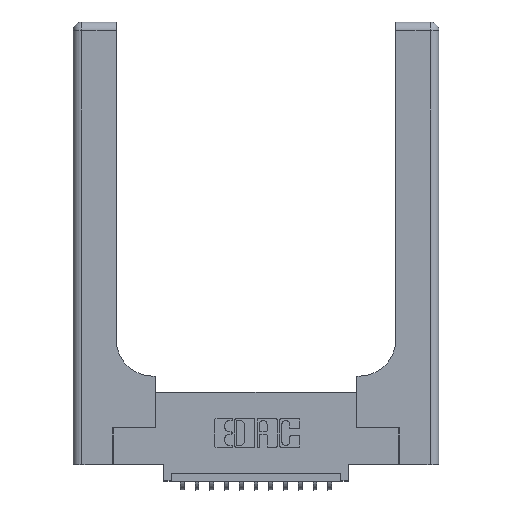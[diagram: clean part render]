
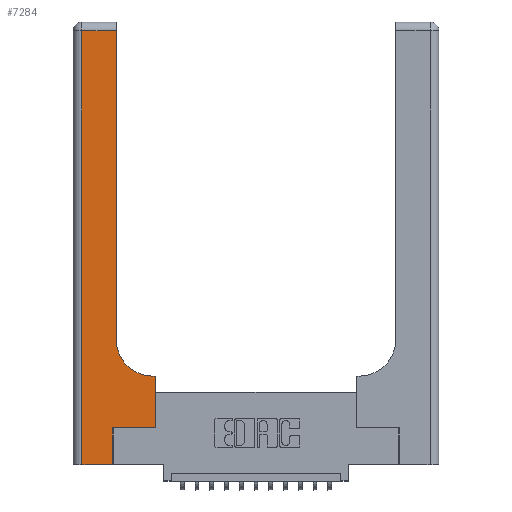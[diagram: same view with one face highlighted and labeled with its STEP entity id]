
A CAD part, top view. The second image highlights one B-rep face of the part: STEP entity #7284.
In plain terms, the highlighted planar face has unit normal (0, 0, 1).
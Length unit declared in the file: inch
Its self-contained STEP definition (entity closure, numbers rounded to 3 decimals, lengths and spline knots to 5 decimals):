
#364 = CARTESIAN_POINT ( 'NONE',  ( 0.5415, 0.6, 0.37 ) ) ;
#785 = LINE ( 'NONE', #7265, #16492 ) ;
#887 = PLANE ( 'NONE',  #12896 ) ;
#1168 = EDGE_CURVE ( 'NONE', #5786, #10817, #5790, .T. ) ;
#1762 = VERTEX_POINT ( 'NONE', #364 ) ;
#1846 = DIRECTION ( 'NONE',  ( -1., 0., 0. ) ) ;
#2134 = CARTESIAN_POINT ( 'NONE',  ( 0., 3., 0.37 ) ) ;
#2148 = VERTEX_POINT ( 'NONE', #14858 ) ;
#2368 = CARTESIAN_POINT ( 'NONE',  ( 0.5585, 0.6, 0.37 ) ) ;
#2928 = DIRECTION ( 'NONE',  ( 1., 0., 0. ) ) ;
#3011 = VERTEX_POINT ( 'NONE', #17585 ) ;
#3127 = ORIENTED_EDGE ( 'NONE', *, *, #14056, .T. ) ;
#3172 = ORIENTED_EDGE ( 'NONE', *, *, #12631, .T. ) ;
#3274 = EDGE_LOOP ( 'NONE', ( #9710, #10301, #8726, #12292, #3172, #3725, #3127, #12026, #11524 ) ) ;
#3385 = DIRECTION ( 'NONE',  ( 0., -1., 0. ) ) ;
#3417 = CARTESIAN_POINT ( 'NONE',  ( 0.2915, 3., 0.37 ) ) ;
#3511 = EDGE_CURVE ( 'NONE', #15576, #5786, #11844, .T. ) ;
#3723 = DIRECTION ( 'NONE',  ( 0., 0., -1. ) ) ;
#3725 = ORIENTED_EDGE ( 'NONE', *, *, #15853, .T. ) ;
#3999 = VECTOR ( 'NONE', #8316, 39.37008 ) ;
#4327 = CARTESIAN_POINT ( 'NONE',  ( 0., 0., 0.37 ) ) ;
#4701 = CARTESIAN_POINT ( 'NONE',  ( 0.2915, 2.94, 0.37 ) ) ;
#4728 = VECTOR ( 'NONE', #15748, 39.37008 ) ;
#5308 = DIRECTION ( 'NONE',  ( 0., 0., -1. ) ) ;
#5344 = VECTOR ( 'NONE', #11607, 39.37008 ) ;
#5596 = LINE ( 'NONE', #11633, #15741 ) ;
#5786 = VERTEX_POINT ( 'NONE', #4701 ) ;
#5790 = LINE ( 'NONE', #8971, #4728 ) ;
#6534 = FACE_OUTER_BOUND ( 'NONE', #3274, .T. ) ;
#6562 = EDGE_CURVE ( 'NONE', #16841, #1762, #785, .T. ) ;
#7040 = VERTEX_POINT ( 'NONE', #7397 ) ;
#7265 = CARTESIAN_POINT ( 'NONE',  ( 0.2915, 0.6, 0.37 ) ) ;
#7284 = ADVANCED_FACE ( 'NONE', ( #6534 ), #887, .F. ) ;
#7299 = LINE ( 'NONE', #4327, #16837 ) ;
#7397 = CARTESIAN_POINT ( 'NONE',  ( 0.269, 0.25, 0.37 ) ) ;
#7401 = CARTESIAN_POINT ( 'NONE',  ( 0.269, 0., 0.37 ) ) ;
#7786 = DIRECTION ( 'NONE',  ( 1., 0., 0. ) ) ;
#8259 = CARTESIAN_POINT ( 'NONE',  ( 0.5585, 0.25, 0.37 ) ) ;
#8316 = DIRECTION ( 'NONE',  ( 0., 1., 0. ) ) ;
#8726 = ORIENTED_EDGE ( 'NONE', *, *, #11644, .T. ) ;
#8971 = CARTESIAN_POINT ( 'NONE',  ( 0., 2.94, 0.37 ) ) ;
#9526 = DIRECTION ( 'NONE',  ( -1., 0., 0. ) ) ;
#9710 = ORIENTED_EDGE ( 'NONE', *, *, #3511, .T. ) ;
#9764 = LINE ( 'NONE', #8259, #3999 ) ;
#10301 = ORIENTED_EDGE ( 'NONE', *, *, #1168, .T. ) ;
#10493 = LINE ( 'NONE', #7401, #5344 ) ;
#10817 = VERTEX_POINT ( 'NONE', #16586 ) ;
#11153 = VECTOR ( 'NONE', #13743, 39.37008 ) ;
#11491 = AXIS2_PLACEMENT_3D ( 'NONE', #13392, #3723, #7786 ) ;
#11511 = EDGE_CURVE ( 'NONE', #2148, #16891, #7299, .T. ) ;
#11524 = ORIENTED_EDGE ( 'NONE', *, *, #15658, .T. ) ;
#11607 = DIRECTION ( 'NONE',  ( 0., 1., 0. ) ) ;
#11633 = CARTESIAN_POINT ( 'NONE',  ( 0.06, 3., 0.37 ) ) ;
#11644 = EDGE_CURVE ( 'NONE', #10817, #2148, #5596, .T. ) ;
#11844 = LINE ( 'NONE', #3417, #14431 ) ;
#12026 = ORIENTED_EDGE ( 'NONE', *, *, #6562, .T. ) ;
#12292 = ORIENTED_EDGE ( 'NONE', *, *, #11511, .T. ) ;
#12631 = EDGE_CURVE ( 'NONE', #16891, #7040, #10493, .T. ) ;
#12896 = AXIS2_PLACEMENT_3D ( 'NONE', #2134, #5308, #9526 ) ;
#13003 = CARTESIAN_POINT ( 'NONE',  ( 0.2915, 0.85, 0.37 ) ) ;
#13392 = CARTESIAN_POINT ( 'NONE',  ( 0.5415, 0.85, 0.37 ) ) ;
#13456 = CARTESIAN_POINT ( 'NONE',  ( 0.269, 0., 0.37 ) ) ;
#13499 = LINE ( 'NONE', #17847, #11153 ) ;
#13717 = CIRCLE ( 'NONE', #11491, 0.25 ) ;
#13743 = DIRECTION ( 'NONE',  ( 1., 0., 0. ) ) ;
#14056 = EDGE_CURVE ( 'NONE', #3011, #16841, #9764, .T. ) ;
#14431 = VECTOR ( 'NONE', #15826, 39.37008 ) ;
#14858 = CARTESIAN_POINT ( 'NONE',  ( 0.06, 0., 0.37 ) ) ;
#15576 = VERTEX_POINT ( 'NONE', #13003 ) ;
#15658 = EDGE_CURVE ( 'NONE', #1762, #15576, #13717, .T. ) ;
#15741 = VECTOR ( 'NONE', #3385, 39.37008 ) ;
#15748 = DIRECTION ( 'NONE',  ( -1., 0., 0. ) ) ;
#15826 = DIRECTION ( 'NONE',  ( 0., 1., 0. ) ) ;
#15853 = EDGE_CURVE ( 'NONE', #7040, #3011, #13499, .T. ) ;
#16492 = VECTOR ( 'NONE', #1846, 39.37008 ) ;
#16586 = CARTESIAN_POINT ( 'NONE',  ( 0.06, 2.94, 0.37 ) ) ;
#16837 = VECTOR ( 'NONE', #2928, 39.37008 ) ;
#16841 = VERTEX_POINT ( 'NONE', #2368 ) ;
#16891 = VERTEX_POINT ( 'NONE', #13456 ) ;
#17585 = CARTESIAN_POINT ( 'NONE',  ( 0.5585, 0.25, 0.37 ) ) ;
#17847 = CARTESIAN_POINT ( 'NONE',  ( 0.269, 0.25, 0.37 ) ) ;
